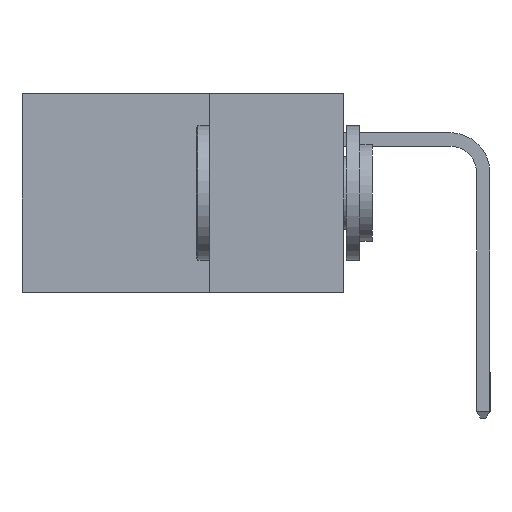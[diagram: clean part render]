
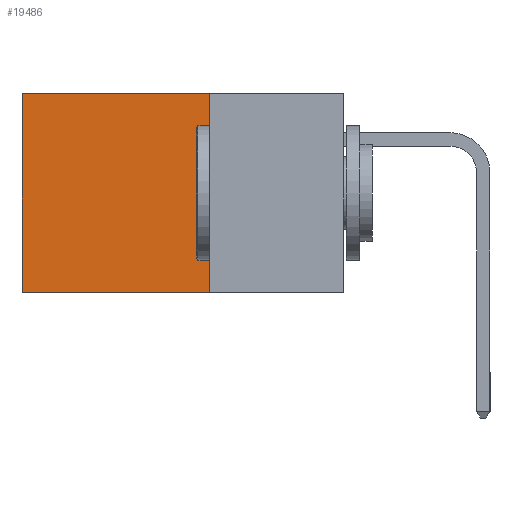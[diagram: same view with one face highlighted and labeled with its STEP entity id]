
A CAD part, left-side view. The second image highlights one B-rep face of the part: STEP entity #19486.
In plain terms, the highlighted planar face has unit normal (-1, 0, 0).
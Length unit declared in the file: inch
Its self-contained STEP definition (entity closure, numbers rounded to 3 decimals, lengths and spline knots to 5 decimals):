
#793 = ORIENTED_EDGE ( 'NONE', *, *, #22230, .F. ) ;
#1136 = ORIENTED_EDGE ( 'NONE', *, *, #21327, .T. ) ;
#1999 = VERTEX_POINT ( 'NONE', #20150 ) ;
#2213 = CARTESIAN_POINT ( 'NONE',  ( 0.298, 0.25, 0. ) ) ;
#4237 = VECTOR ( 'NONE', #26351, 39.37008 ) ;
#4430 = DIRECTION ( 'NONE',  ( 0., 1., 0. ) ) ;
#4590 = LINE ( 'NONE', #26246, #4237 ) ;
#4669 = VECTOR ( 'NONE', #4430, 39.37008 ) ;
#5392 = LINE ( 'NONE', #17926, #4669 ) ;
#8171 = VECTOR ( 'NONE', #14422, 39.37008 ) ;
#8635 = EDGE_LOOP ( 'NONE', ( #22793, #793, #16157, #1136 ) ) ;
#9377 = FACE_OUTER_BOUND ( 'NONE', #8635, .T. ) ;
#10089 = CARTESIAN_POINT ( 'NONE',  ( 0.298, 0.6, -0.37 ) ) ;
#10220 = CARTESIAN_POINT ( 'NONE',  ( 0.298, 0.25, 0. ) ) ;
#11582 = CARTESIAN_POINT ( 'NONE',  ( 0.298, 0.25, -0.37 ) ) ;
#12472 = LINE ( 'NONE', #25746, #8171 ) ;
#13366 = VERTEX_POINT ( 'NONE', #10089 ) ;
#13711 = DIRECTION ( 'NONE',  ( 0., 0., -1. ) ) ;
#13925 = AXIS2_PLACEMENT_3D ( 'NONE', #25432, #27709, #13711 ) ;
#14422 = DIRECTION ( 'NONE',  ( 0., 1., 0. ) ) ;
#16157 = ORIENTED_EDGE ( 'NONE', *, *, #22492, .F. ) ;
#17926 = CARTESIAN_POINT ( 'NONE',  ( 0.298, 0.25, 0. ) ) ;
#18017 = VERTEX_POINT ( 'NONE', #10220 ) ;
#18517 = LINE ( 'NONE', #2213, #23815 ) ;
#19023 = VERTEX_POINT ( 'NONE', #11582 ) ;
#19486 = ADVANCED_FACE ( 'NONE', ( #9377 ), #27311, .F. ) ;
#20150 = CARTESIAN_POINT ( 'NONE',  ( 0.298, 0.6, 0. ) ) ;
#21327 = EDGE_CURVE ( 'NONE', #18017, #1999, #5392, .T. ) ;
#22230 = EDGE_CURVE ( 'NONE', #19023, #13366, #12472, .T. ) ;
#22492 = EDGE_CURVE ( 'NONE', #18017, #19023, #18517, .T. ) ;
#22793 = ORIENTED_EDGE ( 'NONE', *, *, #27816, .T. ) ;
#23815 = VECTOR ( 'NONE', #27288, 39.37008 ) ;
#25432 = CARTESIAN_POINT ( 'NONE',  ( 0.298, 0.25, 0. ) ) ;
#25746 = CARTESIAN_POINT ( 'NONE',  ( 0.298, 0.25, -0.37 ) ) ;
#26246 = CARTESIAN_POINT ( 'NONE',  ( 0.298, 0.6, 0. ) ) ;
#26351 = DIRECTION ( 'NONE',  ( 0., 0., -1. ) ) ;
#27288 = DIRECTION ( 'NONE',  ( 0., 0., -1. ) ) ;
#27311 = PLANE ( 'NONE',  #13925 ) ;
#27709 = DIRECTION ( 'NONE',  ( 1., 0., 0. ) ) ;
#27816 = EDGE_CURVE ( 'NONE', #1999, #13366, #4590, .T. ) ;
